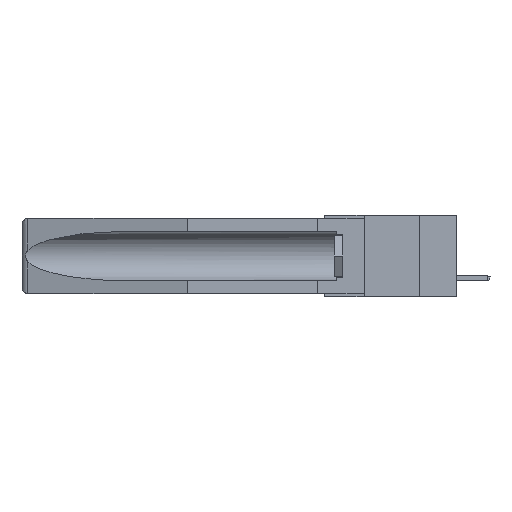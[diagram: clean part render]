
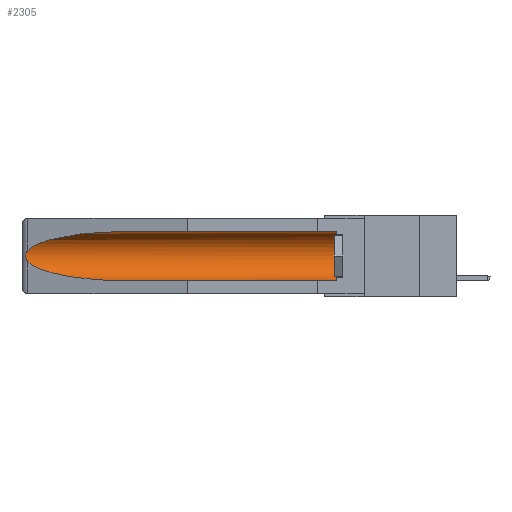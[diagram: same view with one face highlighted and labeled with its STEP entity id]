
A CAD part, left-side view. The second image highlights one B-rep face of the part: STEP entity #2305.
In plain terms, the highlighted cylindrical face has radius 2.857 mm (diameter 5.715 mm), a partial arc.
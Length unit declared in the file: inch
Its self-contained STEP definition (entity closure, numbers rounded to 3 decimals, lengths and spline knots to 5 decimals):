
#329 = AXIS2_PLACEMENT_3D ( 'NONE', #15833, #9068, #20946 ) ;
#420 = LINE ( 'NONE', #3528, #17577 ) ;
#674 = CARTESIAN_POINT ( 'NONE',  ( 0.155, -0.30754, -0.1715 ) ) ;
#944 = CARTESIAN_POINT ( 'NONE',  ( 0.155, 0.126, -0.284 ) ) ;
#1270 = CYLINDRICAL_SURFACE ( 'NONE', #9514, 0.1125 ) ;
#1337 = ORIENTED_EDGE ( 'NONE', *, *, #18036, .F. ) ;
#1472 =( BOUNDED_CURVE ( )  B_SPLINE_CURVE ( 3, ( #20662, #13800, #17339, #10491 ),
 .UNSPECIFIED., .F., .F. ) 
 B_SPLINE_CURVE_WITH_KNOTS ( ( 4, 4 ),
 ( 0.1948, 1.5708 ),
 .UNSPECIFIED. ) 
 CURVE ( )  GEOMETRIC_REPRESENTATION_ITEM ( )  RATIONAL_B_SPLINE_CURVE ( ( 1., 0.848, 0.848, 1. ) ) 
 REPRESENTATION_ITEM ( '' )  );
#1627 = VERTEX_POINT ( 'NONE', #12485 ) ;
#2206 = CARTESIAN_POINT ( 'NONE',  ( 0.26654, 1.53092, -0.15636 ) ) ;
#2305 = ADVANCED_FACE ( 'NONE', ( #19526 ), #1270, .F. ) ;
#2444 = DIRECTION ( 'NONE',  ( 0., 0., 1. ) ) ;
#3127 = EDGE_CURVE ( 'NONE', #10600, #12412, #20138, .T. ) ;
#3128 = CARTESIAN_POINT ( 'NONE',  ( 0.155, 1.07973, -0.059 ) ) ;
#3528 = CARTESIAN_POINT ( 'NONE',  ( 0.155, -0.30754, -0.059 ) ) ;
#3915 = CARTESIAN_POINT ( 'NONE',  ( 0.155, -0.30754, -0.284 ) ) ;
#3933 = CARTESIAN_POINT ( 'NONE',  ( 0.2675, 1.53308, -0.16763 ) ) ;
#4505 = EDGE_CURVE ( 'NONE', #15776, #9519, #13840, .T. ) ;
#4785 = CARTESIAN_POINT ( 'NONE',  ( 0.25451, 1.48313, -0.09465 ) ) ;
#5059 = ORIENTED_EDGE ( 'NONE', *, *, #5075, .T. ) ;
#5075 = EDGE_CURVE ( 'NONE', #9519, #10600, #420, .T. ) ;
#5902 = CARTESIAN_POINT ( 'NONE',  ( 0.26537, 1.52718, -0.19328 ) ) ;
#6022 = CARTESIAN_POINT ( 'NONE',  ( 0.26537, 1.52718, -0.19328 ) ) ;
#7792 = VERTEX_POINT ( 'NONE', #6022 ) ;
#8160 = EDGE_CURVE ( 'NONE', #12412, #7792, #22083, .T. ) ;
#8665 = CARTESIAN_POINT ( 'NONE',  ( 0.155, 1.07973, -0.059 ) ) ;
#8783 = EDGE_CURVE ( 'NONE', #7792, #1627, #1472, .T. ) ;
#9068 = DIRECTION ( 'NONE',  ( 0., -1., 0. ) ) ;
#9208 = CARTESIAN_POINT ( 'NONE',  ( 0.2673, 1.53269, -0.17917 ) ) ;
#9514 = AXIS2_PLACEMENT_3D ( 'NONE', #674, #12746, #2444 ) ;
#9519 = VERTEX_POINT ( 'NONE', #18035 ) ;
#10491 = CARTESIAN_POINT ( 'NONE',  ( 0.155, 1.07973, -0.284 ) ) ;
#10600 = VERTEX_POINT ( 'NONE', #8665 ) ;
#12412 = VERTEX_POINT ( 'NONE', #14293 ) ;
#12485 = CARTESIAN_POINT ( 'NONE',  ( 0.155, 1.07973, -0.284 ) ) ;
#12511 = CARTESIAN_POINT ( 'NONE',  ( 0.26597, 1.52961, -0.15275 ) ) ;
#12746 = DIRECTION ( 'NONE',  ( 0., 1., 0. ) ) ;
#13662 = CARTESIAN_POINT ( 'NONE',  ( 0.26537, 1.52718, -0.14972 ) ) ;
#13800 = CARTESIAN_POINT ( 'NONE',  ( 0.25451, 1.48313, -0.24835 ) ) ;
#13840 = CIRCLE ( 'NONE', #329, 0.1125 ) ;
#14236 = CARTESIAN_POINT ( 'NONE',  ( 0.2673, 1.5327, -0.16383 ) ) ;
#14293 = CARTESIAN_POINT ( 'NONE',  ( 0.26537, 1.52718, -0.14972 ) ) ;
#14597 = CARTESIAN_POINT ( 'NONE',  ( 0.26597, 1.5296, -0.19026 ) ) ;
#14726 = VECTOR ( 'NONE', #21068, 39.37008 ) ;
#14753 = ORIENTED_EDGE ( 'NONE', *, *, #8783, .T. ) ;
#15536 = DIRECTION ( 'NONE',  ( 0., 1., 0. ) ) ;
#15776 = VERTEX_POINT ( 'NONE', #944 ) ;
#15833 = CARTESIAN_POINT ( 'NONE',  ( 0.155, 0.126, -0.1715 ) ) ;
#16506 = ORIENTED_EDGE ( 'NONE', *, *, #8160, .T. ) ;
#16560 = EDGE_LOOP ( 'NONE', ( #17922, #16506, #14753, #1337, #19658, #5059 ) ) ;
#17339 = CARTESIAN_POINT ( 'NONE',  ( 0.21114, 1.30732, -0.284 ) ) ;
#17577 = VECTOR ( 'NONE', #15536, 39.37008 ) ;
#17695 = CARTESIAN_POINT ( 'NONE',  ( 0.2675, 1.53308, -0.17534 ) ) ;
#17922 = ORIENTED_EDGE ( 'NONE', *, *, #3127, .T. ) ;
#18035 = CARTESIAN_POINT ( 'NONE',  ( 0.155, 0.126, -0.059 ) ) ;
#18036 = EDGE_CURVE ( 'NONE', #15776, #1627, #19279, .T. ) ;
#19279 = LINE ( 'NONE', #3915, #14726 ) ;
#19526 = FACE_OUTER_BOUND ( 'NONE', #16560, .T. ) ;
#19658 = ORIENTED_EDGE ( 'NONE', *, *, #4505, .T. ) ;
#20138 =( BOUNDED_CURVE ( )  B_SPLINE_CURVE ( 3, ( #3128, #21875, #4785, #13662 ),
 .UNSPECIFIED., .F., .T. ) 
 B_SPLINE_CURVE_WITH_KNOTS ( ( 4, 4 ),
 ( 4.71239, 6.08839 ),
 .UNSPECIFIED. ) 
 CURVE ( )  GEOMETRIC_REPRESENTATION_ITEM ( )  RATIONAL_B_SPLINE_CURVE ( ( 1., 0.848, 0.848, 1. ) ) 
 REPRESENTATION_ITEM ( '' )  );
#20662 = CARTESIAN_POINT ( 'NONE',  ( 0.26537, 1.52718, -0.19328 ) ) ;
#20946 = DIRECTION ( 'NONE',  ( 0., 0., 1. ) ) ;
#21007 = CARTESIAN_POINT ( 'NONE',  ( 0.26537, 1.52718, -0.14972 ) ) ;
#21068 = DIRECTION ( 'NONE',  ( 0., 1., 0. ) ) ;
#21158 = CARTESIAN_POINT ( 'NONE',  ( 0.26655, 1.53094, -0.18657 ) ) ;
#21875 = CARTESIAN_POINT ( 'NONE',  ( 0.21114, 1.30732, -0.059 ) ) ;
#22083 = B_SPLINE_CURVE_WITH_KNOTS ( 'NONE', 3,
 ( #21007, #12511, #2206, #14236, #3933, #17695, #9208, #21158, #14597, #5902 ),
 .UNSPECIFIED., .F., .F.,
 ( 4, 2, 2, 2, 4 ),
 ( 0., 0.00029, 0.00058, 0.00087, 0.00117 ),
 .UNSPECIFIED. ) ;
